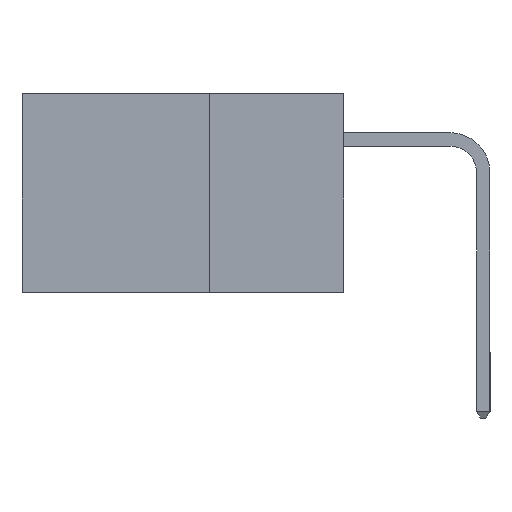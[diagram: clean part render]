
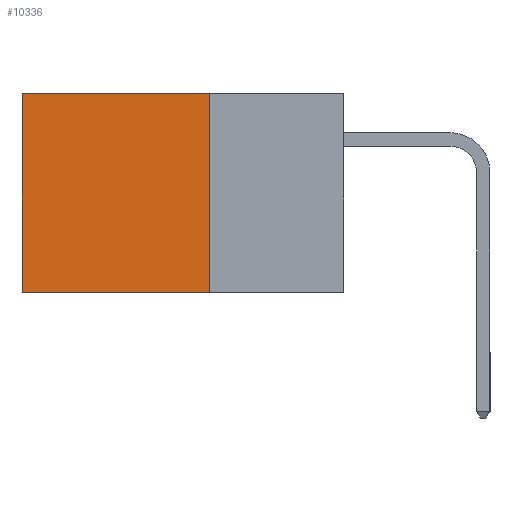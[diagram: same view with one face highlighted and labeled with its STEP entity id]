
A CAD part, left-side view. The second image highlights one B-rep face of the part: STEP entity #10336.
In plain terms, the highlighted planar face has unit normal (-1, 0, 0).
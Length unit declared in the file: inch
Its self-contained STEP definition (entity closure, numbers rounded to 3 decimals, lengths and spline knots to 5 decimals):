
#429 = VECTOR ( 'NONE', #8381, 39.37008 ) ;
#899 = FACE_OUTER_BOUND ( 'NONE', #11362, .T. ) ;
#1691 = DIRECTION ( 'NONE',  ( 0., 0., -1. ) ) ;
#1818 = ORIENTED_EDGE ( 'NONE', *, *, #11449, .F. ) ;
#1965 = ORIENTED_EDGE ( 'NONE', *, *, #8191, .T. ) ;
#2608 = LINE ( 'NONE', #10504, #6993 ) ;
#2966 = CARTESIAN_POINT ( 'NONE',  ( 0.2615, 0.25, -0.37 ) ) ;
#3202 = VECTOR ( 'NONE', #11338, 39.37008 ) ;
#4774 = LINE ( 'NONE', #6670, #429 ) ;
#4927 = EDGE_CURVE ( 'NONE', #5623, #6335, #5936, .T. ) ;
#5367 = DIRECTION ( 'NONE',  ( 0., 0., -1. ) ) ;
#5623 = VERTEX_POINT ( 'NONE', #5657 ) ;
#5657 = CARTESIAN_POINT ( 'NONE',  ( 0.2615, 0.25, 0. ) ) ;
#5936 = LINE ( 'NONE', #6760, #3202 ) ;
#6031 = CARTESIAN_POINT ( 'NONE',  ( 0.2615, 0.25, -0.37 ) ) ;
#6088 = DIRECTION ( 'NONE',  ( 1., 0., 0. ) ) ;
#6335 = VERTEX_POINT ( 'NONE', #8827 ) ;
#6376 = CARTESIAN_POINT ( 'NONE',  ( 0.2615, 0.6, -0.37 ) ) ;
#6569 = DIRECTION ( 'NONE',  ( 0., 1., 0. ) ) ;
#6670 = CARTESIAN_POINT ( 'NONE',  ( 0.2615, 0.25, -0.37 ) ) ;
#6698 = LINE ( 'NONE', #2966, #10340 ) ;
#6760 = CARTESIAN_POINT ( 'NONE',  ( 0.2615, 0.25, 0. ) ) ;
#6895 = CARTESIAN_POINT ( 'NONE',  ( 0.2615, 0.25, -0.37 ) ) ;
#6993 = VECTOR ( 'NONE', #1691, 39.37008 ) ;
#7133 = VERTEX_POINT ( 'NONE', #6895 ) ;
#8191 = EDGE_CURVE ( 'NONE', #6335, #8831, #2608, .T. ) ;
#8381 = DIRECTION ( 'NONE',  ( 0., 0., -1. ) ) ;
#8827 = CARTESIAN_POINT ( 'NONE',  ( 0.2615, 0.6, 0. ) ) ;
#8831 = VERTEX_POINT ( 'NONE', #6376 ) ;
#9274 = ORIENTED_EDGE ( 'NONE', *, *, #4927, .T. ) ;
#9315 = EDGE_CURVE ( 'NONE', #5623, #7133, #4774, .T. ) ;
#9563 = PLANE ( 'NONE',  #11432 ) ;
#10167 = ORIENTED_EDGE ( 'NONE', *, *, #9315, .F. ) ;
#10336 = ADVANCED_FACE ( 'NONE', ( #899 ), #9563, .F. ) ;
#10340 = VECTOR ( 'NONE', #6569, 39.37008 ) ;
#10504 = CARTESIAN_POINT ( 'NONE',  ( 0.2615, 0.6, -0.37 ) ) ;
#11338 = DIRECTION ( 'NONE',  ( 0., 1., 0. ) ) ;
#11362 = EDGE_LOOP ( 'NONE', ( #1965, #1818, #10167, #9274 ) ) ;
#11432 = AXIS2_PLACEMENT_3D ( 'NONE', #6031, #6088, #5367 ) ;
#11449 = EDGE_CURVE ( 'NONE', #7133, #8831, #6698, .T. ) ;
